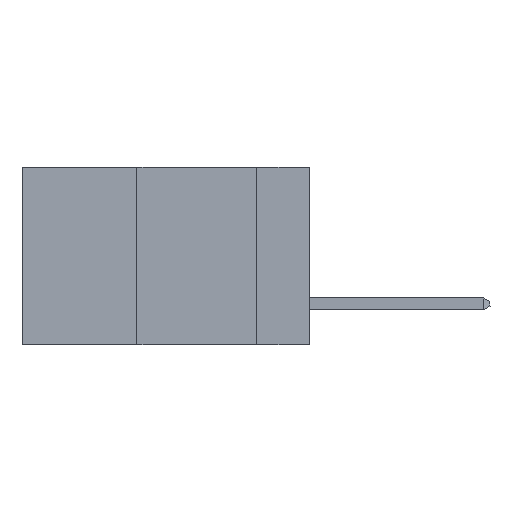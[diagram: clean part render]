
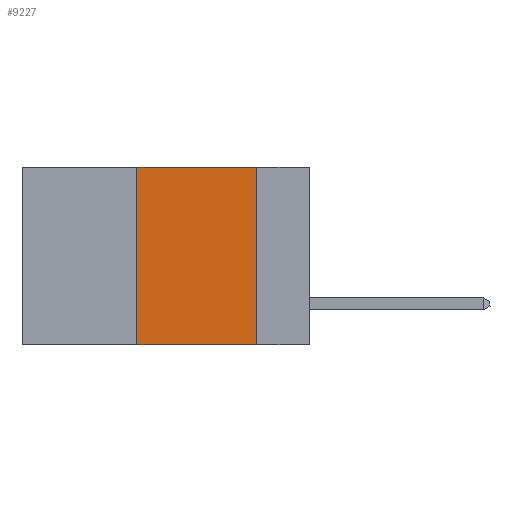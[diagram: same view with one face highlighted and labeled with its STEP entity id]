
A CAD part, left-side view. The second image highlights one B-rep face of the part: STEP entity #9227.
In plain terms, the highlighted planar face has unit normal (-1, 0, 0).
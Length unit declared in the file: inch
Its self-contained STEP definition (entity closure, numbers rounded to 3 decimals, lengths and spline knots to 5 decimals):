
#380 = CARTESIAN_POINT ( 'NONE',  ( 0., 0.11, -0.37 ) ) ;
#1905 = DIRECTION ( 'NONE',  ( 0., 0., -1. ) ) ;
#3079 = EDGE_CURVE ( 'NONE', #30871, #29128, #36044, .T. ) ;
#4111 = LINE ( 'NONE', #25447, #11970 ) ;
#5632 = DIRECTION ( 'NONE',  ( 0., -1., 0. ) ) ;
#6026 = ORIENTED_EDGE ( 'NONE', *, *, #29089, .F. ) ;
#6043 = CARTESIAN_POINT ( 'NONE',  ( 0., 0.6, 0. ) ) ;
#6572 = DIRECTION ( 'NONE',  ( 1., 0., 0. ) ) ;
#8612 = CARTESIAN_POINT ( 'NONE',  ( 0., 0.6, -0.37 ) ) ;
#9227 = ADVANCED_FACE ( 'NONE', ( #13623 ), #29915, .F. ) ;
#9637 = CARTESIAN_POINT ( 'NONE',  ( 0., 0.36, 0. ) ) ;
#9821 = CARTESIAN_POINT ( 'NONE',  ( 0., 0.36, 0. ) ) ;
#10069 = LINE ( 'NONE', #6043, #16079 ) ;
#11970 = VECTOR ( 'NONE', #1905, 39.37008 ) ;
#12211 = CARTESIAN_POINT ( 'NONE',  ( 0., 0.11, 0. ) ) ;
#12780 = VECTOR ( 'NONE', #5632, 39.37008 ) ;
#13464 = LINE ( 'NONE', #9637, #36716 ) ;
#13623 = FACE_OUTER_BOUND ( 'NONE', #18001, .T. ) ;
#16079 = VECTOR ( 'NONE', #20717, 39.37008 ) ;
#18001 = EDGE_LOOP ( 'NONE', ( #34412, #6026, #33076, #18505 ) ) ;
#18505 = ORIENTED_EDGE ( 'NONE', *, *, #3079, .T. ) ;
#20717 = DIRECTION ( 'NONE',  ( 0., -1., 0. ) ) ;
#24076 = CARTESIAN_POINT ( 'NONE',  ( 0., 0.6, 0. ) ) ;
#24288 = DIRECTION ( 'NONE',  ( 0., 0., 1. ) ) ;
#25447 = CARTESIAN_POINT ( 'NONE',  ( 0., 0.11, 0. ) ) ;
#27139 = DIRECTION ( 'NONE',  ( 0., 0., -1. ) ) ;
#27481 = EDGE_CURVE ( 'NONE', #33223, #29128, #4111, .T. ) ;
#29089 = EDGE_CURVE ( 'NONE', #37388, #33223, #10069, .T. ) ;
#29128 = VERTEX_POINT ( 'NONE', #380 ) ;
#29915 = PLANE ( 'NONE',  #31639 ) ;
#30871 = VERTEX_POINT ( 'NONE', #32054 ) ;
#31639 = AXIS2_PLACEMENT_3D ( 'NONE', #24076, #6572, #27139 ) ;
#32054 = CARTESIAN_POINT ( 'NONE',  ( 0., 0.36, -0.37 ) ) ;
#33076 = ORIENTED_EDGE ( 'NONE', *, *, #33291, .F. ) ;
#33223 = VERTEX_POINT ( 'NONE', #12211 ) ;
#33291 = EDGE_CURVE ( 'NONE', #30871, #37388, #13464, .T. ) ;
#34412 = ORIENTED_EDGE ( 'NONE', *, *, #27481, .F. ) ;
#36044 = LINE ( 'NONE', #8612, #12780 ) ;
#36716 = VECTOR ( 'NONE', #24288, 39.37008 ) ;
#37388 = VERTEX_POINT ( 'NONE', #9821 ) ;
